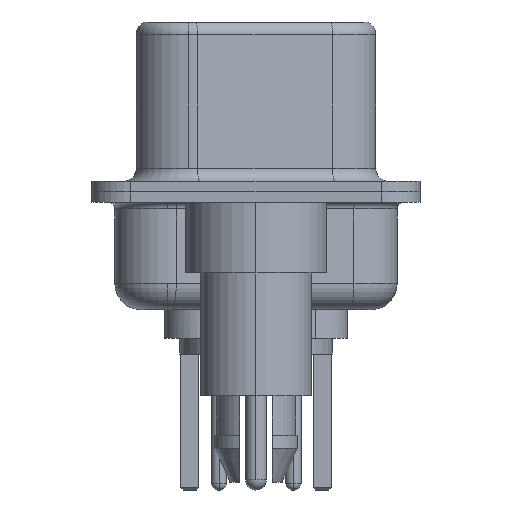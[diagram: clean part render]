
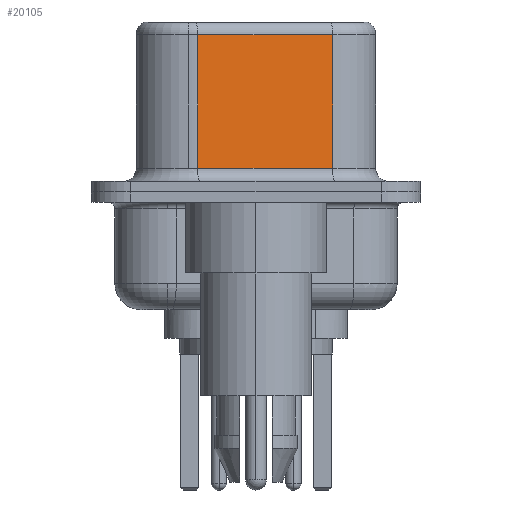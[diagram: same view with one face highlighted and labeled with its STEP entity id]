
A CAD part, left-side view. The second image highlights one B-rep face of the part: STEP entity #20105.
In plain terms, the highlighted planar face has unit normal (-0.985, -0.174, 0).
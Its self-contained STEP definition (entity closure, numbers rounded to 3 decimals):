
#339 = LINE ( 'NONE', #4257, #23130 ) ;
#382 = VERTEX_POINT ( 'NONE', #12548 ) ;
#2815 = DIRECTION ( 'NONE',  ( 0.985, 0.174, 0. ) ) ;
#2903 = LINE ( 'NONE', #23045, #21475 ) ;
#4257 = CARTESIAN_POINT ( 'NONE',  ( 4.565, -2.927, 6.02 ) ) ;
#5336 = VECTOR ( 'NONE', #10740, 1000. ) ;
#5899 = CARTESIAN_POINT ( 'NONE',  ( 3.655, 2.233, 0.9 ) ) ;
#5903 = EDGE_LOOP ( 'NONE', ( #13704, #14567, #11773, #20000 ) ) ;
#6087 = DIRECTION ( 'NONE',  ( -0.174, 0.985, 0. ) ) ;
#7132 = CARTESIAN_POINT ( 'NONE',  ( 3.655, 2.233, 6.02 ) ) ;
#7825 = EDGE_CURVE ( 'NONE', #21856, #8329, #11385, .T. ) ;
#7938 = VERTEX_POINT ( 'NONE', #10318 ) ;
#8329 = VERTEX_POINT ( 'NONE', #5899 ) ;
#10273 = VECTOR ( 'NONE', #11334, 1000. ) ;
#10318 = CARTESIAN_POINT ( 'NONE',  ( 4.565, -2.927, 0.9 ) ) ;
#10407 = EDGE_CURVE ( 'NONE', #382, #21856, #339, .T. ) ;
#10740 = DIRECTION ( 'NONE',  ( 0., 0., -1. ) ) ;
#11305 = CARTESIAN_POINT ( 'NONE',  ( 3.655, 2.233, 6.52 ) ) ;
#11334 = DIRECTION ( 'NONE',  ( 0., 0., -1. ) ) ;
#11385 = LINE ( 'NONE', #11305, #10273 ) ;
#11773 = ORIENTED_EDGE ( 'NONE', *, *, #7825, .T. ) ;
#12548 = CARTESIAN_POINT ( 'NONE',  ( 4.565, -2.927, 6.02 ) ) ;
#13624 = PLANE ( 'NONE',  #16097 ) ;
#13704 = ORIENTED_EDGE ( 'NONE', *, *, #20961, .F. ) ;
#14567 = ORIENTED_EDGE ( 'NONE', *, *, #10407, .T. ) ;
#15328 = CARTESIAN_POINT ( 'NONE',  ( 4.565, -2.927, 6.52 ) ) ;
#15404 = DIRECTION ( 'NONE',  ( -0.174, 0.985, 0. ) ) ;
#16070 = CARTESIAN_POINT ( 'NONE',  ( 4.565, -2.927, 6.52 ) ) ;
#16097 = AXIS2_PLACEMENT_3D ( 'NONE', #15328, #2815, #15404 ) ;
#17310 = EDGE_CURVE ( 'NONE', #8329, #7938, #2903, .T. ) ;
#17634 = DIRECTION ( 'NONE',  ( 0.174, -0.985, 0. ) ) ;
#17687 = FACE_OUTER_BOUND ( 'NONE', #5903, .T. ) ;
#19654 = LINE ( 'NONE', #16070, #5336 ) ;
#20000 = ORIENTED_EDGE ( 'NONE', *, *, #17310, .T. ) ;
#20105 = ADVANCED_FACE ( 'NONE', ( #17687 ), #13624, .F. ) ;
#20961 = EDGE_CURVE ( 'NONE', #382, #7938, #19654, .T. ) ;
#21475 = VECTOR ( 'NONE', #17634, 1000. ) ;
#21856 = VERTEX_POINT ( 'NONE', #7132 ) ;
#23045 = CARTESIAN_POINT ( 'NONE',  ( 4.565, -2.927, 0.9 ) ) ;
#23130 = VECTOR ( 'NONE', #6087, 1000. ) ;
